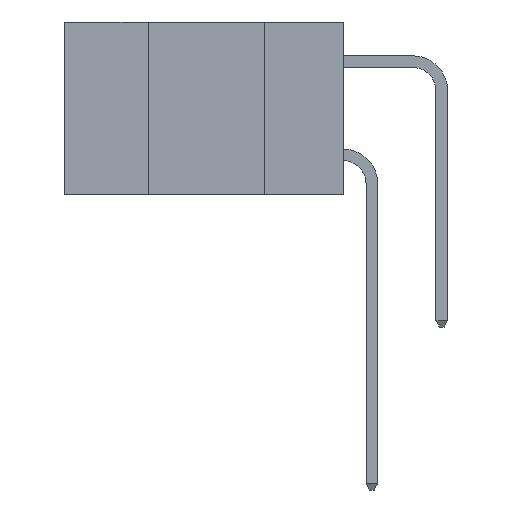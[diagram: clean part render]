
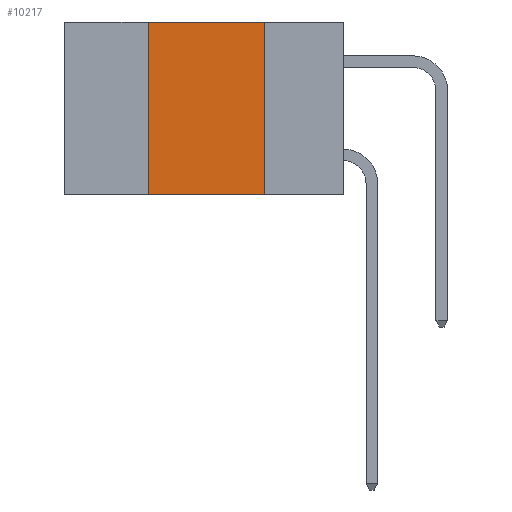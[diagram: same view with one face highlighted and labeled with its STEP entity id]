
A CAD part, left-side view. The second image highlights one B-rep face of the part: STEP entity #10217.
In plain terms, the highlighted planar face has unit normal (-1, 0, 0).
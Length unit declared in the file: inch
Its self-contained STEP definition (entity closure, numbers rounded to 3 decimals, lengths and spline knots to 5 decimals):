
#1277 = VECTOR ( 'NONE', #14492, 39.37008 ) ;
#2164 = EDGE_LOOP ( 'NONE', ( #26898, #16132, #21873, #16833 ) ) ;
#2882 = EDGE_CURVE ( 'NONE', #4056, #27748, #20147, .T. ) ;
#3274 = DIRECTION ( 'NONE',  ( 1., 0., 0. ) ) ;
#4056 = VERTEX_POINT ( 'NONE', #17798 ) ;
#4099 = FACE_OUTER_BOUND ( 'NONE', #2164, .T. ) ;
#4643 = DIRECTION ( 'NONE',  ( 0., -1., 0. ) ) ;
#4961 = AXIS2_PLACEMENT_3D ( 'NONE', #18366, #3274, #18455 ) ;
#5079 = CARTESIAN_POINT ( 'NONE',  ( 0., 0.6, 0. ) ) ;
#5298 = DIRECTION ( 'NONE',  ( 0., -1., 0. ) ) ;
#5810 = EDGE_CURVE ( 'NONE', #27748, #9116, #18633, .T. ) ;
#7292 = CARTESIAN_POINT ( 'NONE',  ( 0., 0.42, -0.37 ) ) ;
#8614 = VECTOR ( 'NONE', #4643, 39.37008 ) ;
#9116 = VERTEX_POINT ( 'NONE', #23124 ) ;
#10217 = ADVANCED_FACE ( 'NONE', ( #4099 ), #16299, .F. ) ;
#11064 = VECTOR ( 'NONE', #26758, 39.37008 ) ;
#11067 = CARTESIAN_POINT ( 'NONE',  ( 0., 0.17, 0. ) ) ;
#11663 = CARTESIAN_POINT ( 'NONE',  ( 0., 0.6, -0.37 ) ) ;
#12018 = EDGE_CURVE ( 'NONE', #15983, #4056, #12421, .T. ) ;
#12421 = LINE ( 'NONE', #7292, #11064 ) ;
#12619 = VECTOR ( 'NONE', #5298, 39.37008 ) ;
#12834 = CARTESIAN_POINT ( 'NONE',  ( 0., 0.42, -0.37 ) ) ;
#14492 = DIRECTION ( 'NONE',  ( 0., 0., -1. ) ) ;
#14686 = CARTESIAN_POINT ( 'NONE',  ( 0., 0.17, -0.37 ) ) ;
#15983 = VERTEX_POINT ( 'NONE', #12834 ) ;
#16132 = ORIENTED_EDGE ( 'NONE', *, *, #2882, .F. ) ;
#16299 = PLANE ( 'NONE',  #4961 ) ;
#16833 = ORIENTED_EDGE ( 'NONE', *, *, #20863, .T. ) ;
#17798 = CARTESIAN_POINT ( 'NONE',  ( 0., 0.42, 0. ) ) ;
#18366 = CARTESIAN_POINT ( 'NONE',  ( 0., 0.6, 0. ) ) ;
#18455 = DIRECTION ( 'NONE',  ( 0., 0., -1. ) ) ;
#18633 = LINE ( 'NONE', #14686, #1277 ) ;
#20147 = LINE ( 'NONE', #5079, #8614 ) ;
#20863 = EDGE_CURVE ( 'NONE', #15983, #9116, #24063, .T. ) ;
#21873 = ORIENTED_EDGE ( 'NONE', *, *, #12018, .F. ) ;
#23124 = CARTESIAN_POINT ( 'NONE',  ( 0., 0.17, -0.37 ) ) ;
#24063 = LINE ( 'NONE', #11663, #12619 ) ;
#26758 = DIRECTION ( 'NONE',  ( 0., 0., 1. ) ) ;
#26898 = ORIENTED_EDGE ( 'NONE', *, *, #5810, .F. ) ;
#27748 = VERTEX_POINT ( 'NONE', #11067 ) ;
